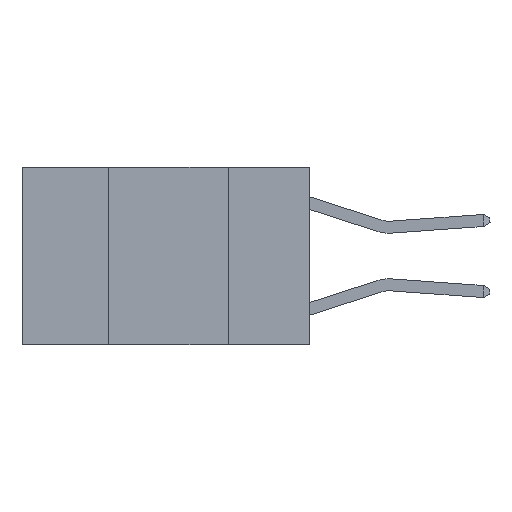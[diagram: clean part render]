
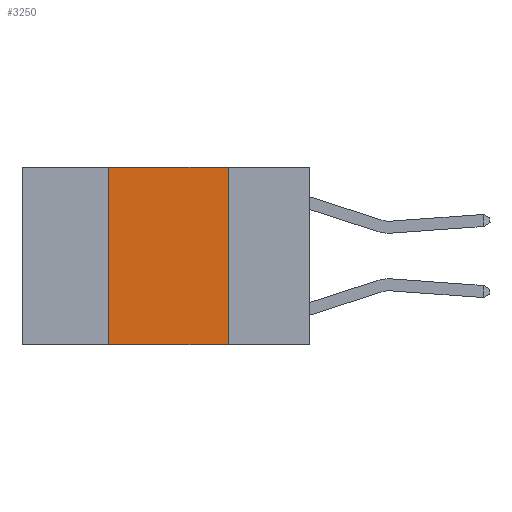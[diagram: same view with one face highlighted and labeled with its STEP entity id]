
A CAD part, left-side view. The second image highlights one B-rep face of the part: STEP entity #3250.
In plain terms, the highlighted planar face has unit normal (-1, 0, 0).
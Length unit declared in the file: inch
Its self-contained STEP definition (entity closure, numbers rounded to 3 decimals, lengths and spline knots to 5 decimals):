
#190 = AXIS2_PLACEMENT_3D ( 'NONE', #7721, #2721, #8417 ) ;
#1268 = CARTESIAN_POINT ( 'NONE',  ( 0., 0.6, -0.37 ) ) ;
#1274 = VERTEX_POINT ( 'NONE', #4837 ) ;
#1584 = VECTOR ( 'NONE', #9065, 39.37008 ) ;
#1811 = PLANE ( 'NONE',  #190 ) ;
#1899 = VERTEX_POINT ( 'NONE', #9905 ) ;
#2014 = VERTEX_POINT ( 'NONE', #3618 ) ;
#2194 = DIRECTION ( 'NONE',  ( 0., -1., 0. ) ) ;
#2393 = VERTEX_POINT ( 'NONE', #6250 ) ;
#2681 = VECTOR ( 'NONE', #3888, 39.37008 ) ;
#2721 = DIRECTION ( 'NONE',  ( 1., 0., 0. ) ) ;
#2726 = CARTESIAN_POINT ( 'NONE',  ( 0., 0.17, 0. ) ) ;
#2775 = VECTOR ( 'NONE', #2194, 39.37008 ) ;
#3250 = ADVANCED_FACE ( 'NONE', ( #5983 ), #1811, .F. ) ;
#3606 = EDGE_LOOP ( 'NONE', ( #7349, #6877, #8122, #7505 ) ) ;
#3618 = CARTESIAN_POINT ( 'NONE',  ( 0., 0.17, -0.37 ) ) ;
#3888 = DIRECTION ( 'NONE',  ( 0., 0., 1. ) ) ;
#3989 = EDGE_CURVE ( 'NONE', #1274, #2014, #9287, .T. ) ;
#4837 = CARTESIAN_POINT ( 'NONE',  ( 0., 0.42, -0.37 ) ) ;
#5264 = EDGE_CURVE ( 'NONE', #2393, #1899, #8347, .T. ) ;
#5360 = EDGE_CURVE ( 'NONE', #1899, #2014, #9974, .T. ) ;
#5983 = FACE_OUTER_BOUND ( 'NONE', #3606, .T. ) ;
#6173 = VECTOR ( 'NONE', #6834, 39.37008 ) ;
#6250 = CARTESIAN_POINT ( 'NONE',  ( 0., 0.42, 0. ) ) ;
#6628 = EDGE_CURVE ( 'NONE', #1274, #2393, #7194, .T. ) ;
#6834 = DIRECTION ( 'NONE',  ( 0., -1., 0. ) ) ;
#6877 = ORIENTED_EDGE ( 'NONE', *, *, #5264, .F. ) ;
#7194 = LINE ( 'NONE', #9281, #2681 ) ;
#7349 = ORIENTED_EDGE ( 'NONE', *, *, #5360, .F. ) ;
#7500 = CARTESIAN_POINT ( 'NONE',  ( 0., 0.6, 0. ) ) ;
#7505 = ORIENTED_EDGE ( 'NONE', *, *, #3989, .T. ) ;
#7721 = CARTESIAN_POINT ( 'NONE',  ( 0., 0.6, 0. ) ) ;
#8122 = ORIENTED_EDGE ( 'NONE', *, *, #6628, .F. ) ;
#8347 = LINE ( 'NONE', #7500, #6173 ) ;
#8417 = DIRECTION ( 'NONE',  ( 0., 0., -1. ) ) ;
#9065 = DIRECTION ( 'NONE',  ( 0., 0., -1. ) ) ;
#9281 = CARTESIAN_POINT ( 'NONE',  ( 0., 0.42, 0. ) ) ;
#9287 = LINE ( 'NONE', #1268, #2775 ) ;
#9905 = CARTESIAN_POINT ( 'NONE',  ( 0., 0.17, 0. ) ) ;
#9974 = LINE ( 'NONE', #2726, #1584 ) ;
